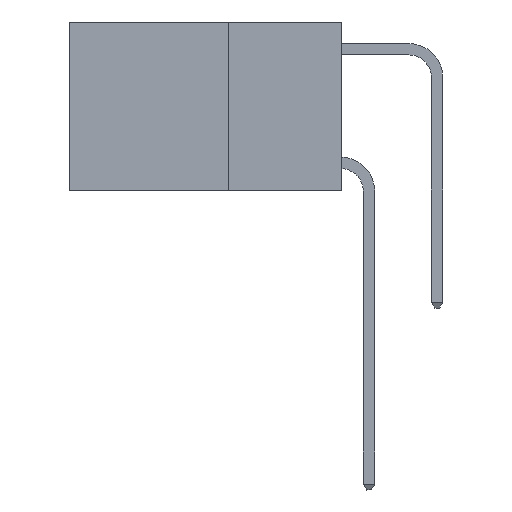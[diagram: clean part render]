
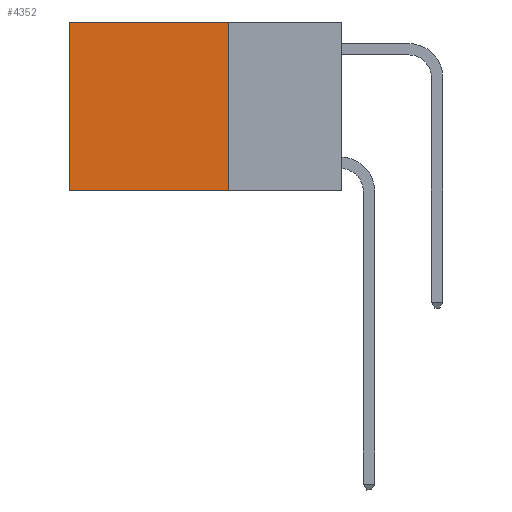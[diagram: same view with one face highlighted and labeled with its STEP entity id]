
A CAD part, left-side view. The second image highlights one B-rep face of the part: STEP entity #4352.
In plain terms, the highlighted planar face has unit normal (-1, 0, 0).
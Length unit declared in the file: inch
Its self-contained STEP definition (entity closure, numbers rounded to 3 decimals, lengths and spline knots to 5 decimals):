
#602 = VECTOR ( 'NONE', #2866, 39.37008 ) ;
#788 = CARTESIAN_POINT ( 'NONE',  ( 0.2625, 0.6, 0. ) ) ;
#1618 = EDGE_CURVE ( 'NONE', #15145, #14482, #4683, .T. ) ;
#1645 = EDGE_CURVE ( 'NONE', #15145, #8618, #3924, .T. ) ;
#1781 = LINE ( 'NONE', #788, #10299 ) ;
#1811 = VECTOR ( 'NONE', #5137, 39.37008 ) ;
#2866 = DIRECTION ( 'NONE',  ( 0., 0., -1. ) ) ;
#3463 = FACE_OUTER_BOUND ( 'NONE', #8255, .T. ) ;
#3924 = LINE ( 'NONE', #5190, #602 ) ;
#4007 = CARTESIAN_POINT ( 'NONE',  ( 0.2625, 0.25, -0.37 ) ) ;
#4352 = ADVANCED_FACE ( 'NONE', ( #3463 ), #9536, .F. ) ;
#4683 = LINE ( 'NONE', #12411, #1811 ) ;
#5137 = DIRECTION ( 'NONE',  ( 0., 1., 0. ) ) ;
#5187 = CARTESIAN_POINT ( 'NONE',  ( 0.2625, 0.6, 0. ) ) ;
#5190 = CARTESIAN_POINT ( 'NONE',  ( 0.2625, 0.25, 0. ) ) ;
#5518 = DIRECTION ( 'NONE',  ( 0., 1., 0. ) ) ;
#5964 = DIRECTION ( 'NONE',  ( 1., 0., 0. ) ) ;
#7070 = ORIENTED_EDGE ( 'NONE', *, *, #10287, .F. ) ;
#7534 = ORIENTED_EDGE ( 'NONE', *, *, #1618, .T. ) ;
#8238 = AXIS2_PLACEMENT_3D ( 'NONE', #13204, #5964, #14429 ) ;
#8255 = EDGE_LOOP ( 'NONE', ( #9970, #7070, #10742, #7534 ) ) ;
#8276 = LINE ( 'NONE', #12787, #11547 ) ;
#8618 = VERTEX_POINT ( 'NONE', #4007 ) ;
#9414 = CARTESIAN_POINT ( 'NONE',  ( 0.2625, 0.6, -0.37 ) ) ;
#9536 = PLANE ( 'NONE',  #8238 ) ;
#9962 = CARTESIAN_POINT ( 'NONE',  ( 0.2625, 0.25, 0. ) ) ;
#9970 = ORIENTED_EDGE ( 'NONE', *, *, #15493, .T. ) ;
#10287 = EDGE_CURVE ( 'NONE', #8618, #11608, #8276, .T. ) ;
#10299 = VECTOR ( 'NONE', #11824, 39.37008 ) ;
#10742 = ORIENTED_EDGE ( 'NONE', *, *, #1645, .F. ) ;
#11547 = VECTOR ( 'NONE', #5518, 39.37008 ) ;
#11608 = VERTEX_POINT ( 'NONE', #9414 ) ;
#11824 = DIRECTION ( 'NONE',  ( 0., 0., -1. ) ) ;
#12411 = CARTESIAN_POINT ( 'NONE',  ( 0.2625, 0.25, 0. ) ) ;
#12787 = CARTESIAN_POINT ( 'NONE',  ( 0.2625, 0.25, -0.37 ) ) ;
#13204 = CARTESIAN_POINT ( 'NONE',  ( 0.2625, 0.25, 0. ) ) ;
#14429 = DIRECTION ( 'NONE',  ( 0., 0., -1. ) ) ;
#14482 = VERTEX_POINT ( 'NONE', #5187 ) ;
#15145 = VERTEX_POINT ( 'NONE', #9962 ) ;
#15493 = EDGE_CURVE ( 'NONE', #14482, #11608, #1781, .T. ) ;
